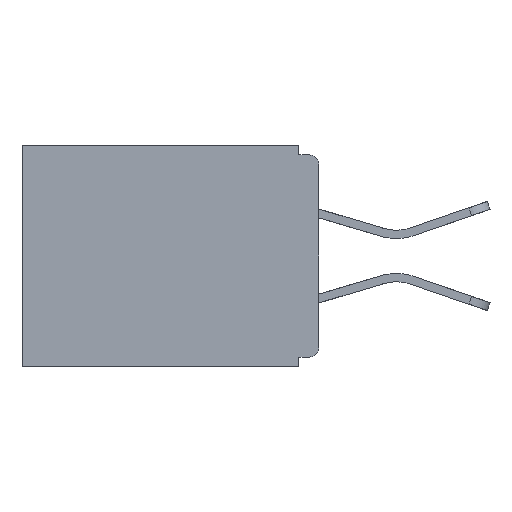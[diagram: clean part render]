
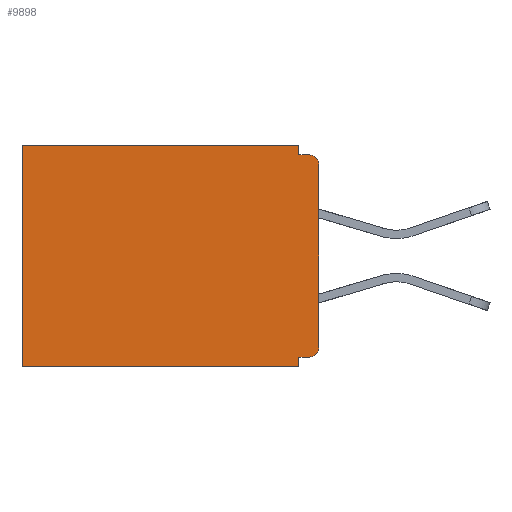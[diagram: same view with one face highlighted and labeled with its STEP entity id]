
A CAD part, left-side view. The second image highlights one B-rep face of the part: STEP entity #9898.
In plain terms, the highlighted planar face has unit normal (-1, 0, 0).
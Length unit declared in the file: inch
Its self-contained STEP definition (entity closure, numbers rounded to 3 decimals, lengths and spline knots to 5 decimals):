
#79 = AXIS2_PLACEMENT_3D ( 'NONE', #3475, #25281, #27252 ) ;
#187 = LINE ( 'NONE', #658, #23484 ) ;
#544 = CARTESIAN_POINT ( 'NONE',  ( 0.298, 0.031, -0.343 ) ) ;
#658 = CARTESIAN_POINT ( 'NONE',  ( 0.298, 0., 0. ) ) ;
#799 = DIRECTION ( 'NONE',  ( 0., 0., -1. ) ) ;
#823 = VERTEX_POINT ( 'NONE', #3273 ) ;
#1253 = CARTESIAN_POINT ( 'NONE',  ( 0.298, 0.031, 0. ) ) ;
#1748 = FACE_OUTER_BOUND ( 'NONE', #10580, .T. ) ;
#2071 = CARTESIAN_POINT ( 'NONE',  ( 0.298, 0., -0.343 ) ) ;
#2472 = AXIS2_PLACEMENT_3D ( 'NONE', #8757, #16926, #23631 ) ;
#2961 = VERTEX_POINT ( 'NONE', #544 ) ;
#3273 = CARTESIAN_POINT ( 'NONE',  ( 0.298, 0.46, -0.343 ) ) ;
#3369 = EDGE_CURVE ( 'NONE', #15392, #5283, #7334, .T. ) ;
#3475 = CARTESIAN_POINT ( 'NONE',  ( 0.298, 0., 0. ) ) ;
#3518 = CARTESIAN_POINT ( 'NONE',  ( 0.298, 0.46, 0. ) ) ;
#3591 = EDGE_CURVE ( 'NONE', #9902, #17644, #14238, .T. ) ;
#4031 = CARTESIAN_POINT ( 'NONE',  ( 0.298, 0.031, -0.343 ) ) ;
#4097 = LINE ( 'NONE', #4255, #26022 ) ;
#4255 = CARTESIAN_POINT ( 'NONE',  ( 0.298, 0., -0.328 ) ) ;
#4715 = CARTESIAN_POINT ( 'NONE',  ( 0.298, 0.015, -0.313 ) ) ;
#4993 = DIRECTION ( 'NONE',  ( 0., 0., -1. ) ) ;
#5283 = VERTEX_POINT ( 'NONE', #12361 ) ;
#5496 = VERTEX_POINT ( 'NONE', #11776 ) ;
#5664 = EDGE_CURVE ( 'NONE', #5496, #823, #21290, .T. ) ;
#5910 = ORIENTED_EDGE ( 'NONE', *, *, #3591, .F. ) ;
#6390 = EDGE_CURVE ( 'NONE', #7566, #2961, #10285, .T. ) ;
#6875 = CARTESIAN_POINT ( 'NONE',  ( 0.298, 0.031, -0.015 ) ) ;
#7331 = DIRECTION ( 'NONE',  ( 0., 1., 0. ) ) ;
#7334 = LINE ( 'NONE', #9415, #19303 ) ;
#7566 = VERTEX_POINT ( 'NONE', #8053 ) ;
#7905 = DIRECTION ( 'NONE',  ( 0., 0., -1. ) ) ;
#7941 = EDGE_CURVE ( 'NONE', #9902, #5496, #187, .T. ) ;
#8053 = CARTESIAN_POINT ( 'NONE',  ( 0.298, 0.031, -0.328 ) ) ;
#8757 = CARTESIAN_POINT ( 'NONE',  ( 0.298, 0.015, -0.03 ) ) ;
#9239 = ORIENTED_EDGE ( 'NONE', *, *, #12168, .T. ) ;
#9415 = CARTESIAN_POINT ( 'NONE',  ( 0.298, 0., 0. ) ) ;
#9561 = ORIENTED_EDGE ( 'NONE', *, *, #26344, .T. ) ;
#9755 = ORIENTED_EDGE ( 'NONE', *, *, #13874, .F. ) ;
#9778 = CARTESIAN_POINT ( 'NONE',  ( 0.298, 0.031, -0.343 ) ) ;
#9847 = DIRECTION ( 'NONE',  ( 0., 0., -1. ) ) ;
#9898 = ADVANCED_FACE ( 'NONE', ( #1748 ), #16174, .F. ) ;
#9902 = VERTEX_POINT ( 'NONE', #1253 ) ;
#9958 = EDGE_CURVE ( 'NONE', #2961, #823, #15679, .T. ) ;
#10285 = LINE ( 'NONE', #9778, #19920 ) ;
#10580 = EDGE_LOOP ( 'NONE', ( #9239, #25608, #5910, #18120, #24447, #16344, #27540, #9755, #9561, #11477 ) ) ;
#10902 = VECTOR ( 'NONE', #17256, 39.37008 ) ;
#11477 = ORIENTED_EDGE ( 'NONE', *, *, #3369, .F. ) ;
#11776 = CARTESIAN_POINT ( 'NONE',  ( 0.298, 0.46, 0. ) ) ;
#12168 = EDGE_CURVE ( 'NONE', #15392, #20769, #22740, .T. ) ;
#12361 = CARTESIAN_POINT ( 'NONE',  ( 0.298, 0., -0.313 ) ) ;
#12521 = DIRECTION ( 'NONE',  ( 0., 1., 0. ) ) ;
#13874 = EDGE_CURVE ( 'NONE', #20478, #7566, #4097, .T. ) ;
#14238 = LINE ( 'NONE', #4031, #15262 ) ;
#15184 = CIRCLE ( 'NONE', #21775, 0.015 ) ;
#15262 = VECTOR ( 'NONE', #27440, 39.37008 ) ;
#15392 = VERTEX_POINT ( 'NONE', #25424 ) ;
#15679 = LINE ( 'NONE', #2071, #18696 ) ;
#16174 = PLANE ( 'NONE',  #79 ) ;
#16344 = ORIENTED_EDGE ( 'NONE', *, *, #9958, .F. ) ;
#16926 = DIRECTION ( 'NONE',  ( -1., 0., 0. ) ) ;
#17256 = DIRECTION ( 'NONE',  ( 0., -1., 0. ) ) ;
#17644 = VERTEX_POINT ( 'NONE', #6875 ) ;
#17701 = EDGE_CURVE ( 'NONE', #17644, #20769, #22224, .T. ) ;
#18120 = ORIENTED_EDGE ( 'NONE', *, *, #7941, .T. ) ;
#18696 = VECTOR ( 'NONE', #12521, 39.37008 ) ;
#19303 = VECTOR ( 'NONE', #4993, 39.37008 ) ;
#19920 = VECTOR ( 'NONE', #7905, 39.37008 ) ;
#20298 = CARTESIAN_POINT ( 'NONE',  ( 0.298, 0.015, -0.015 ) ) ;
#20478 = VERTEX_POINT ( 'NONE', #22573 ) ;
#20769 = VERTEX_POINT ( 'NONE', #20298 ) ;
#20969 = VECTOR ( 'NONE', #9847, 39.37008 ) ;
#21290 = LINE ( 'NONE', #3518, #20969 ) ;
#21752 = CARTESIAN_POINT ( 'NONE',  ( 0.298, 0., -0.015 ) ) ;
#21775 = AXIS2_PLACEMENT_3D ( 'NONE', #4715, #25959, #799 ) ;
#22224 = LINE ( 'NONE', #21752, #10902 ) ;
#22573 = CARTESIAN_POINT ( 'NONE',  ( 0.298, 0.015, -0.328 ) ) ;
#22740 = CIRCLE ( 'NONE', #2472, 0.015 ) ;
#23484 = VECTOR ( 'NONE', #7331, 39.37008 ) ;
#23485 = DIRECTION ( 'NONE',  ( 0., 1., 0. ) ) ;
#23631 = DIRECTION ( 'NONE',  ( 0., 0., -1. ) ) ;
#24447 = ORIENTED_EDGE ( 'NONE', *, *, #5664, .T. ) ;
#25281 = DIRECTION ( 'NONE',  ( 1., 0., 0. ) ) ;
#25424 = CARTESIAN_POINT ( 'NONE',  ( 0.298, 0., -0.03 ) ) ;
#25608 = ORIENTED_EDGE ( 'NONE', *, *, #17701, .F. ) ;
#25959 = DIRECTION ( 'NONE',  ( -1., 0., 0. ) ) ;
#26022 = VECTOR ( 'NONE', #23485, 39.37008 ) ;
#26344 = EDGE_CURVE ( 'NONE', #20478, #5283, #15184, .T. ) ;
#27252 = DIRECTION ( 'NONE',  ( 0., 0., -1. ) ) ;
#27440 = DIRECTION ( 'NONE',  ( 0., 0., -1. ) ) ;
#27540 = ORIENTED_EDGE ( 'NONE', *, *, #6390, .F. ) ;
